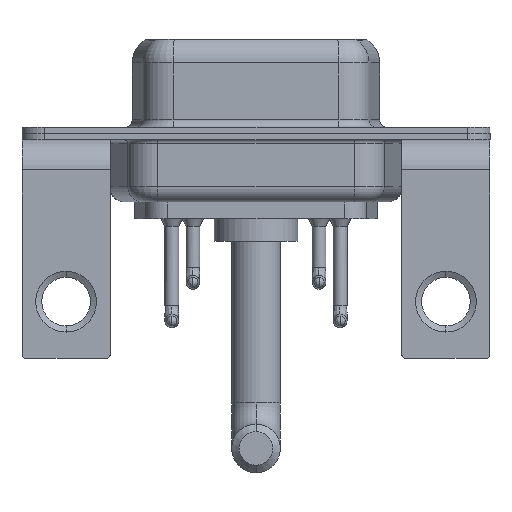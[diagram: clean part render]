
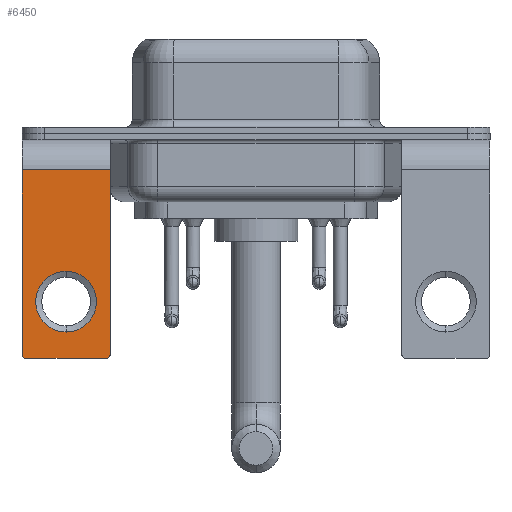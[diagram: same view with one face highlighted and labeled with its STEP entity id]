
A CAD part, front view. The second image highlights one B-rep face of the part: STEP entity #6450.
In plain terms, the highlighted planar face has unit normal (0, -1, 0).
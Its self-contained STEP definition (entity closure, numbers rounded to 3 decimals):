
#211 = DIRECTION ( 'NONE',  ( 0., 0., 1. ) ) ;
#346 = CARTESIAN_POINT ( 'NONE',  ( 2.9, -6.25, -2.4 ) ) ;
#378 = LINE ( 'NONE', #5745, #8745 ) ;
#400 = DIRECTION ( 'NONE',  ( 0., -1., 0. ) ) ;
#834 = FACE_OUTER_BOUND ( 'NONE', #14916, .T. ) ;
#902 = DIRECTION ( 'NONE',  ( 0., 0., 1. ) ) ;
#947 = CARTESIAN_POINT ( 'NONE',  ( 2.9, -6.25, -2.4 ) ) ;
#1143 = EDGE_CURVE ( 'NONE', #3075, #7620, #11574, .T. ) ;
#1226 = AXIS2_PLACEMENT_3D ( 'NONE', #10759, #8158, #211 ) ;
#1691 = EDGE_CURVE ( 'NONE', #3901, #14825, #2609, .T. ) ;
#1809 = ORIENTED_EDGE ( 'NONE', *, *, #10968, .T. ) ;
#1963 = CARTESIAN_POINT ( 'NONE',  ( -2.65, -6.25, -14.55 ) ) ;
#2049 = FACE_BOUND ( 'NONE', #7428, .T. ) ;
#2217 = EDGE_CURVE ( 'NONE', #4427, #15428, #2858, .T. ) ;
#2285 = CARTESIAN_POINT ( 'NONE',  ( 2.9, -6.25, -2.4 ) ) ;
#2609 = CIRCLE ( 'NONE', #1226, 2. ) ;
#2858 = CIRCLE ( 'NONE', #12540, 0.25 ) ;
#3075 = VERTEX_POINT ( 'NONE', #4840 ) ;
#3335 = PLANE ( 'NONE',  #13918 ) ;
#3528 = DIRECTION ( 'NONE',  ( -1., 0., 0. ) ) ;
#3804 = CARTESIAN_POINT ( 'NONE',  ( -2.65, -6.25, -14.8 ) ) ;
#3874 = DIRECTION ( 'NONE',  ( 0., 0., -1. ) ) ;
#3901 = VERTEX_POINT ( 'NONE', #6262 ) ;
#4332 = LINE ( 'NONE', #346, #16851 ) ;
#4427 = VERTEX_POINT ( 'NONE', #14104 ) ;
#4732 = CARTESIAN_POINT ( 'NONE',  ( 2.65, -6.25, -14.55 ) ) ;
#4794 = ORIENTED_EDGE ( 'NONE', *, *, #2217, .T. ) ;
#4840 = CARTESIAN_POINT ( 'NONE',  ( 2.9, -6.25, -2.4 ) ) ;
#4892 = DIRECTION ( 'NONE',  ( 0., -1., 0. ) ) ;
#5441 = ORIENTED_EDGE ( 'NONE', *, *, #1691, .T. ) ;
#5745 = CARTESIAN_POINT ( 'NONE',  ( 2.9, -6.25, -14.8 ) ) ;
#5968 = ORIENTED_EDGE ( 'NONE', *, *, #1143, .T. ) ;
#5991 = VERTEX_POINT ( 'NONE', #13499 ) ;
#6069 = VECTOR ( 'NONE', #3874, 1000. ) ;
#6262 = CARTESIAN_POINT ( 'NONE',  ( 0., -6.25, -13.07 ) ) ;
#6305 = AXIS2_PLACEMENT_3D ( 'NONE', #1963, #400, #11207 ) ;
#6356 = ORIENTED_EDGE ( 'NONE', *, *, #7113, .F. ) ;
#6450 = ADVANCED_FACE ( 'NONE', ( #2049, #834 ), #3335, .F. ) ;
#7098 = CIRCLE ( 'NONE', #10683, 2. ) ;
#7113 = EDGE_CURVE ( 'NONE', #4427, #13015, #378, .T. ) ;
#7428 = EDGE_LOOP ( 'NONE', ( #5441, #9808 ) ) ;
#7620 = VERTEX_POINT ( 'NONE', #13501 ) ;
#8012 = CARTESIAN_POINT ( 'NONE',  ( 2.9, -6.25, -14.55 ) ) ;
#8158 = DIRECTION ( 'NONE',  ( 0., 1., 0. ) ) ;
#8745 = VECTOR ( 'NONE', #13431, 1000. ) ;
#8760 = DIRECTION ( 'NONE',  ( 0., 1., 0. ) ) ;
#9053 = CIRCLE ( 'NONE', #6305, 0.25 ) ;
#9063 = LINE ( 'NONE', #15648, #6069 ) ;
#9574 = EDGE_CURVE ( 'NONE', #14825, #3901, #7098, .T. ) ;
#9808 = ORIENTED_EDGE ( 'NONE', *, *, #9574, .T. ) ;
#10215 = DIRECTION ( 'NONE',  ( 0., 1., 0. ) ) ;
#10683 = AXIS2_PLACEMENT_3D ( 'NONE', #16869, #10215, #902 ) ;
#10759 = CARTESIAN_POINT ( 'NONE',  ( 0., -6.25, -11.07 ) ) ;
#10968 = EDGE_CURVE ( 'NONE', #5991, #13015, #9053, .T. ) ;
#11207 = DIRECTION ( 'NONE',  ( 0., 0., 1. ) ) ;
#11532 = ORIENTED_EDGE ( 'NONE', *, *, #15133, .F. ) ;
#11574 = LINE ( 'NONE', #947, #13661 ) ;
#12540 = AXIS2_PLACEMENT_3D ( 'NONE', #4732, #4892, #12845 ) ;
#12596 = DIRECTION ( 'NONE',  ( 0., 0., 1. ) ) ;
#12807 = CARTESIAN_POINT ( 'NONE',  ( 0., -6.25, -9.07 ) ) ;
#12845 = DIRECTION ( 'NONE',  ( 0., 0., 1. ) ) ;
#13015 = VERTEX_POINT ( 'NONE', #3804 ) ;
#13431 = DIRECTION ( 'NONE',  ( -1., 0., 0. ) ) ;
#13499 = CARTESIAN_POINT ( 'NONE',  ( -2.9, -6.25, -14.55 ) ) ;
#13501 = CARTESIAN_POINT ( 'NONE',  ( -2.9, -6.25, -2.4 ) ) ;
#13661 = VECTOR ( 'NONE', #3528, 1000. ) ;
#13746 = EDGE_CURVE ( 'NONE', #7620, #5991, #9063, .T. ) ;
#13918 = AXIS2_PLACEMENT_3D ( 'NONE', #2285, #8760, #12596 ) ;
#14104 = CARTESIAN_POINT ( 'NONE',  ( 2.65, -6.25, -14.8 ) ) ;
#14379 = ORIENTED_EDGE ( 'NONE', *, *, #13746, .T. ) ;
#14825 = VERTEX_POINT ( 'NONE', #12807 ) ;
#14916 = EDGE_LOOP ( 'NONE', ( #14379, #1809, #6356, #4794, #11532, #5968 ) ) ;
#15060 = DIRECTION ( 'NONE',  ( 0., 0., -1. ) ) ;
#15133 = EDGE_CURVE ( 'NONE', #3075, #15428, #4332, .T. ) ;
#15428 = VERTEX_POINT ( 'NONE', #8012 ) ;
#15648 = CARTESIAN_POINT ( 'NONE',  ( -2.9, -6.25, -2.4 ) ) ;
#16851 = VECTOR ( 'NONE', #15060, 1000. ) ;
#16869 = CARTESIAN_POINT ( 'NONE',  ( 0., -6.25, -11.07 ) ) ;
